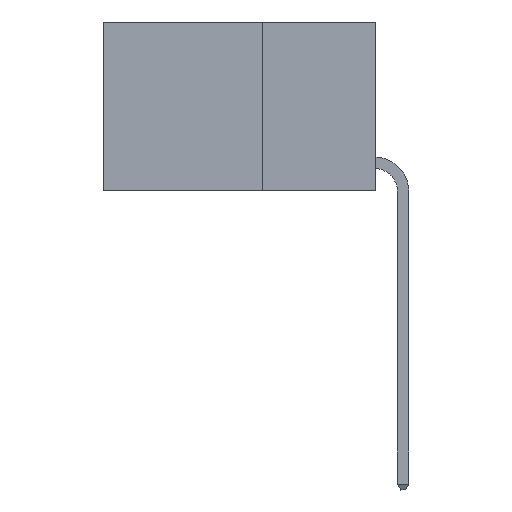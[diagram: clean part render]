
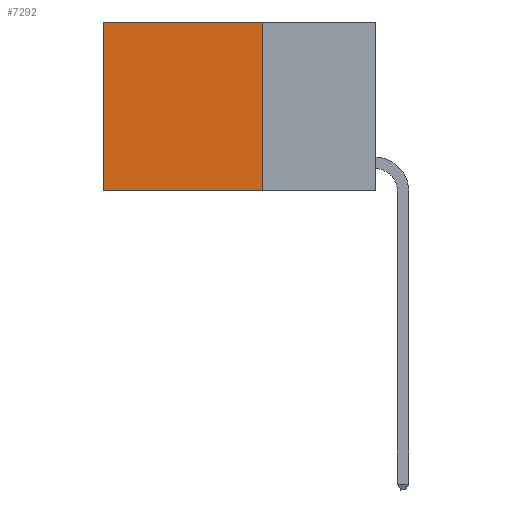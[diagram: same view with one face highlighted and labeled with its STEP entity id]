
A CAD part, left-side view. The second image highlights one B-rep face of the part: STEP entity #7292.
In plain terms, the highlighted planar face has unit normal (-1, 0, 0).
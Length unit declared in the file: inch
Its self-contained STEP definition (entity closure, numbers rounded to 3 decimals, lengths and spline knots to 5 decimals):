
#165 = CARTESIAN_POINT ( 'NONE',  ( 0.2625, 0.25, -0.37 ) ) ;
#554 = ORIENTED_EDGE ( 'NONE', *, *, #8060, .F. ) ;
#601 = CARTESIAN_POINT ( 'NONE',  ( 0.2625, 0.25, 0. ) ) ;
#756 = CARTESIAN_POINT ( 'NONE',  ( 0.2625, 0.6, -0.37 ) ) ;
#1152 = VERTEX_POINT ( 'NONE', #2379 ) ;
#1268 = CARTESIAN_POINT ( 'NONE',  ( 0.2625, 0.25, 0. ) ) ;
#2012 = LINE ( 'NONE', #14115, #7899 ) ;
#2115 = PLANE ( 'NONE',  #14197 ) ;
#2379 = CARTESIAN_POINT ( 'NONE',  ( 0.2625, 0.25, 0. ) ) ;
#2456 = DIRECTION ( 'NONE',  ( 0., 0., -1. ) ) ;
#3312 = DIRECTION ( 'NONE',  ( 0., 0., -1. ) ) ;
#4081 = ORIENTED_EDGE ( 'NONE', *, *, #4857, .T. ) ;
#4857 = EDGE_CURVE ( 'NONE', #5406, #5451, #2012, .T. ) ;
#5406 = VERTEX_POINT ( 'NONE', #9939 ) ;
#5447 = VECTOR ( 'NONE', #2456, 39.37008 ) ;
#5451 = VERTEX_POINT ( 'NONE', #756 ) ;
#6062 = DIRECTION ( 'NONE',  ( 0., 1., 0. ) ) ;
#7292 = ADVANCED_FACE ( 'NONE', ( #13636 ), #2115, .F. ) ;
#7498 = EDGE_CURVE ( 'NONE', #9890, #5451, #7643, .T. ) ;
#7643 = LINE ( 'NONE', #165, #12903 ) ;
#7899 = VECTOR ( 'NONE', #12233, 39.37008 ) ;
#8060 = EDGE_CURVE ( 'NONE', #1152, #9890, #13924, .T. ) ;
#8316 = EDGE_CURVE ( 'NONE', #1152, #5406, #11196, .T. ) ;
#9497 = ORIENTED_EDGE ( 'NONE', *, *, #8316, .T. ) ;
#9729 = CARTESIAN_POINT ( 'NONE',  ( 0.2625, 0.25, -0.37 ) ) ;
#9890 = VERTEX_POINT ( 'NONE', #9729 ) ;
#9939 = CARTESIAN_POINT ( 'NONE',  ( 0.2625, 0.6, 0. ) ) ;
#10189 = DIRECTION ( 'NONE',  ( 1., 0., 0. ) ) ;
#10706 = EDGE_LOOP ( 'NONE', ( #4081, #13927, #554, #9497 ) ) ;
#11196 = LINE ( 'NONE', #601, #11520 ) ;
#11520 = VECTOR ( 'NONE', #13841, 39.37008 ) ;
#12233 = DIRECTION ( 'NONE',  ( 0., 0., -1. ) ) ;
#12903 = VECTOR ( 'NONE', #6062, 39.37008 ) ;
#13636 = FACE_OUTER_BOUND ( 'NONE', #10706, .T. ) ;
#13841 = DIRECTION ( 'NONE',  ( 0., 1., 0. ) ) ;
#13924 = LINE ( 'NONE', #1268, #5447 ) ;
#13927 = ORIENTED_EDGE ( 'NONE', *, *, #7498, .F. ) ;
#14115 = CARTESIAN_POINT ( 'NONE',  ( 0.2625, 0.6, 0. ) ) ;
#14120 = CARTESIAN_POINT ( 'NONE',  ( 0.2625, 0.25, 0. ) ) ;
#14197 = AXIS2_PLACEMENT_3D ( 'NONE', #14120, #10189, #3312 ) ;
